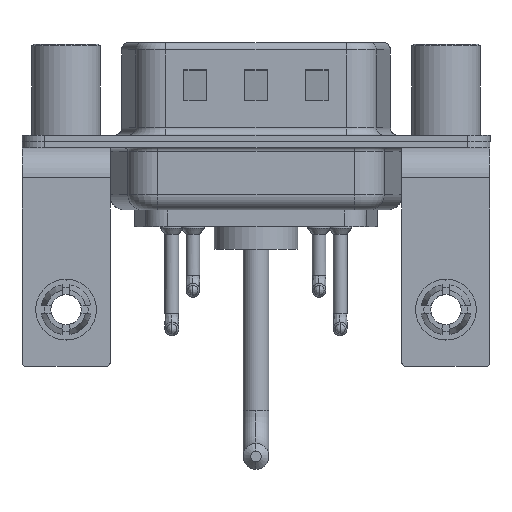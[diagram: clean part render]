
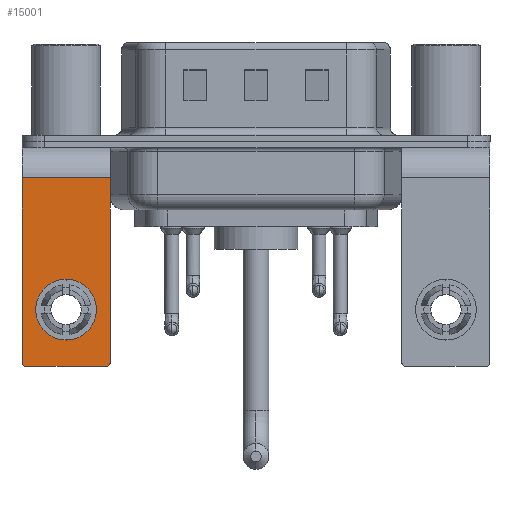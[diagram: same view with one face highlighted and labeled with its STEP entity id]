
A CAD part, front view. The second image highlights one B-rep face of the part: STEP entity #15001.
In plain terms, the highlighted planar face has unit normal (0, -1, 0).
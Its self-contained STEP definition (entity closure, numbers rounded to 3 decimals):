
#686 = DIRECTION ( 'NONE',  ( -1., 0., 0. ) ) ;
#953 = DIRECTION ( 'NONE',  ( 0., 0., 1. ) ) ;
#989 = CARTESIAN_POINT ( 'NONE',  ( -2.65, -6.25, -14.55 ) ) ;
#1335 = DIRECTION ( 'NONE',  ( 0., -1., 0. ) ) ;
#1383 = DIRECTION ( 'NONE',  ( 0., -1., 0. ) ) ;
#1636 = EDGE_LOOP ( 'NONE', ( #16946, #5318 ) ) ;
#2041 = VECTOR ( 'NONE', #14034, 1000. ) ;
#2320 = EDGE_CURVE ( 'NONE', #11326, #16630, #18763, .T. ) ;
#2519 = LINE ( 'NONE', #18242, #17748 ) ;
#2735 = EDGE_CURVE ( 'NONE', #16630, #11326, #4905, .T. ) ;
#3088 = CARTESIAN_POINT ( 'NONE',  ( 2.9, -6.25, -2.4 ) ) ;
#3212 = EDGE_CURVE ( 'NONE', #3957, #7670, #22825, .T. ) ;
#3504 = CARTESIAN_POINT ( 'NONE',  ( -2.9, -6.25, -2.4 ) ) ;
#3530 = EDGE_CURVE ( 'NONE', #4738, #10615, #6397, .T. ) ;
#3641 = DIRECTION ( 'NONE',  ( 0., 0., 1. ) ) ;
#3854 = CARTESIAN_POINT ( 'NONE',  ( 2.65, -6.25, -14.8 ) ) ;
#3957 = VERTEX_POINT ( 'NONE', #14520 ) ;
#4279 = CARTESIAN_POINT ( 'NONE',  ( 0., -6.25, -9.07 ) ) ;
#4328 = VECTOR ( 'NONE', #8616, 1000. ) ;
#4589 = VERTEX_POINT ( 'NONE', #3854 ) ;
#4738 = VERTEX_POINT ( 'NONE', #3088 ) ;
#4784 = ORIENTED_EDGE ( 'NONE', *, *, #21758, .T. ) ;
#4905 = CIRCLE ( 'NONE', #17810, 2. ) ;
#4973 = DIRECTION ( 'NONE',  ( 0., 1., 0. ) ) ;
#4978 = PLANE ( 'NONE',  #13911 ) ;
#5318 = ORIENTED_EDGE ( 'NONE', *, *, #2735, .T. ) ;
#5483 = AXIS2_PLACEMENT_3D ( 'NONE', #989, #1335, #9893 ) ;
#5558 = DIRECTION ( 'NONE',  ( 0., 0., -1. ) ) ;
#6397 = LINE ( 'NONE', #10431, #16699 ) ;
#6711 = DIRECTION ( 'NONE',  ( 0., 0., 1. ) ) ;
#7670 = VERTEX_POINT ( 'NONE', #15472 ) ;
#8234 = DIRECTION ( 'NONE',  ( 0., 0., 1. ) ) ;
#8567 = FACE_OUTER_BOUND ( 'NONE', #13003, .T. ) ;
#8616 = DIRECTION ( 'NONE',  ( -1., 0., 0. ) ) ;
#8750 = CARTESIAN_POINT ( 'NONE',  ( 0., -6.25, -13.07 ) ) ;
#9149 = CIRCLE ( 'NONE', #17274, 0.25 ) ;
#9473 = EDGE_CURVE ( 'NONE', #4589, #14083, #2519, .T. ) ;
#9710 = ORIENTED_EDGE ( 'NONE', *, *, #18046, .T. ) ;
#9893 = DIRECTION ( 'NONE',  ( 0., 0., 1. ) ) ;
#10431 = CARTESIAN_POINT ( 'NONE',  ( 2.9, -6.25, -2.4 ) ) ;
#10615 = VERTEX_POINT ( 'NONE', #12855 ) ;
#11326 = VERTEX_POINT ( 'NONE', #8750 ) ;
#11885 = CARTESIAN_POINT ( 'NONE',  ( -2.65, -6.25, -14.8 ) ) ;
#11916 = DIRECTION ( 'NONE',  ( 0., 1., 0. ) ) ;
#12397 = LINE ( 'NONE', #19570, #4328 ) ;
#12855 = CARTESIAN_POINT ( 'NONE',  ( 2.9, -6.25, -14.55 ) ) ;
#12867 = CIRCLE ( 'NONE', #5483, 0.25 ) ;
#13003 = EDGE_LOOP ( 'NONE', ( #18187, #4784, #22621, #9710, #16666, #20503 ) ) ;
#13593 = AXIS2_PLACEMENT_3D ( 'NONE', #22667, #4973, #953 ) ;
#13911 = AXIS2_PLACEMENT_3D ( 'NONE', #17216, #11916, #8234 ) ;
#14034 = DIRECTION ( 'NONE',  ( 0., 0., -1. ) ) ;
#14083 = VERTEX_POINT ( 'NONE', #11885 ) ;
#14285 = CARTESIAN_POINT ( 'NONE',  ( 0., -6.25, -11.07 ) ) ;
#14520 = CARTESIAN_POINT ( 'NONE',  ( -2.9, -6.25, -2.4 ) ) ;
#15001 = ADVANCED_FACE ( 'NONE', ( #20810, #8567 ), #4978, .F. ) ;
#15472 = CARTESIAN_POINT ( 'NONE',  ( -2.9, -6.25, -14.55 ) ) ;
#16630 = VERTEX_POINT ( 'NONE', #4279 ) ;
#16666 = ORIENTED_EDGE ( 'NONE', *, *, #3530, .F. ) ;
#16699 = VECTOR ( 'NONE', #5558, 1000. ) ;
#16946 = ORIENTED_EDGE ( 'NONE', *, *, #2320, .T. ) ;
#17108 = EDGE_CURVE ( 'NONE', #4738, #3957, #12397, .T. ) ;
#17206 = CARTESIAN_POINT ( 'NONE',  ( 2.65, -6.25, -14.55 ) ) ;
#17216 = CARTESIAN_POINT ( 'NONE',  ( 2.9, -6.25, -2.4 ) ) ;
#17274 = AXIS2_PLACEMENT_3D ( 'NONE', #17206, #1383, #6711 ) ;
#17748 = VECTOR ( 'NONE', #686, 1000. ) ;
#17810 = AXIS2_PLACEMENT_3D ( 'NONE', #14285, #19376, #3641 ) ;
#18046 = EDGE_CURVE ( 'NONE', #4589, #10615, #9149, .T. ) ;
#18187 = ORIENTED_EDGE ( 'NONE', *, *, #3212, .T. ) ;
#18242 = CARTESIAN_POINT ( 'NONE',  ( 2.9, -6.25, -14.8 ) ) ;
#18763 = CIRCLE ( 'NONE', #13593, 2. ) ;
#19376 = DIRECTION ( 'NONE',  ( 0., 1., 0. ) ) ;
#19570 = CARTESIAN_POINT ( 'NONE',  ( 2.9, -6.25, -2.4 ) ) ;
#20503 = ORIENTED_EDGE ( 'NONE', *, *, #17108, .T. ) ;
#20810 = FACE_BOUND ( 'NONE', #1636, .T. ) ;
#21758 = EDGE_CURVE ( 'NONE', #7670, #14083, #12867, .T. ) ;
#22621 = ORIENTED_EDGE ( 'NONE', *, *, #9473, .F. ) ;
#22667 = CARTESIAN_POINT ( 'NONE',  ( 0., -6.25, -11.07 ) ) ;
#22825 = LINE ( 'NONE', #3504, #2041 ) ;
